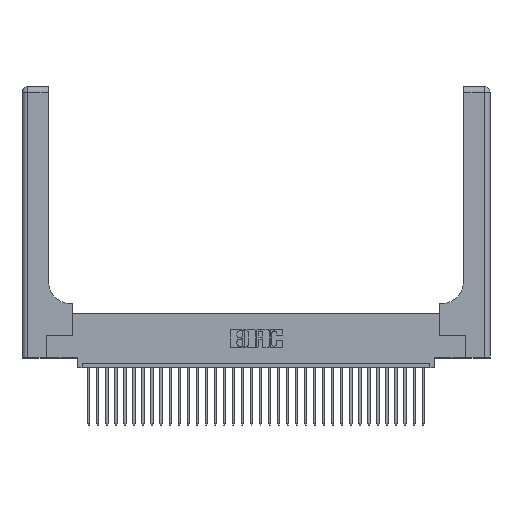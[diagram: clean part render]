
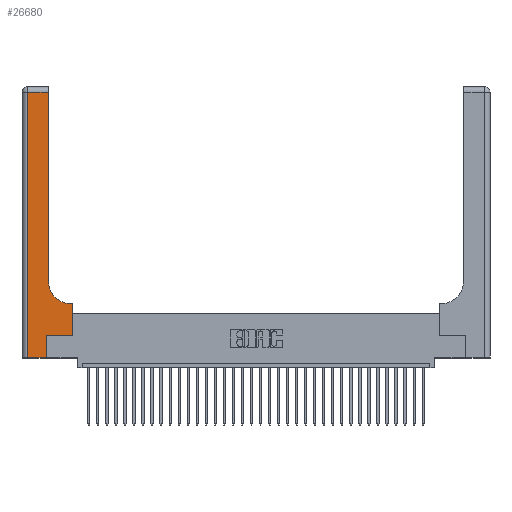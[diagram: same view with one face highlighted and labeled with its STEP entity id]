
A CAD part, top view. The second image highlights one B-rep face of the part: STEP entity #26680.
In plain terms, the highlighted planar face has unit normal (0, 0, 1).
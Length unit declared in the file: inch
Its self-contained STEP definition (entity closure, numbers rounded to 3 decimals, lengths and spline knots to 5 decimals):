
#269 = ORIENTED_EDGE ( 'NONE', *, *, #11622, .T. ) ;
#581 = CARTESIAN_POINT ( 'NONE',  ( 0.2915, 0.85, 0.37 ) ) ;
#1344 = LINE ( 'NONE', #22579, #9231 ) ;
#1752 = VERTEX_POINT ( 'NONE', #25194 ) ;
#2163 = CARTESIAN_POINT ( 'NONE',  ( 0.2915, 3., 0.37 ) ) ;
#3003 = EDGE_CURVE ( 'NONE', #11323, #3056, #8525, .T. ) ;
#3056 = VERTEX_POINT ( 'NONE', #7794 ) ;
#3455 = CARTESIAN_POINT ( 'NONE',  ( 0.269, 0.25, 0.37 ) ) ;
#3712 = DIRECTION ( 'NONE',  ( 1., 0., 0. ) ) ;
#4756 = EDGE_CURVE ( 'NONE', #32752, #34467, #1344, .T. ) ;
#4982 = LINE ( 'NONE', #12663, #9131 ) ;
#5082 = CARTESIAN_POINT ( 'NONE',  ( 0.5415, 0.6, 0.37 ) ) ;
#5227 = VECTOR ( 'NONE', #7631, 39.37008 ) ;
#5939 = VECTOR ( 'NONE', #33972, 39.37008 ) ;
#6462 = CARTESIAN_POINT ( 'NONE',  ( 0.06, 0., 0.37 ) ) ;
#6854 = DIRECTION ( 'NONE',  ( 0., 0., -1. ) ) ;
#6968 = LINE ( 'NONE', #7161, #7808 ) ;
#7161 = CARTESIAN_POINT ( 'NONE',  ( 0.5585, 0.25, 0.37 ) ) ;
#7584 = CARTESIAN_POINT ( 'NONE',  ( 0.2915, 0.6, 0.37 ) ) ;
#7631 = DIRECTION ( 'NONE',  ( 1., 0., 0. ) ) ;
#7659 = LINE ( 'NONE', #7584, #5939 ) ;
#7794 = CARTESIAN_POINT ( 'NONE',  ( 0.269, 0., 0.37 ) ) ;
#7808 = VECTOR ( 'NONE', #12409, 39.37008 ) ;
#8030 = ORIENTED_EDGE ( 'NONE', *, *, #11778, .T. ) ;
#8525 = LINE ( 'NONE', #12889, #5227 ) ;
#8648 = EDGE_CURVE ( 'NONE', #1752, #29394, #6968, .T. ) ;
#9131 = VECTOR ( 'NONE', #25964, 39.37008 ) ;
#9231 = VECTOR ( 'NONE', #12066, 39.37008 ) ;
#11323 = VERTEX_POINT ( 'NONE', #6462 ) ;
#11380 = VECTOR ( 'NONE', #23519, 39.37008 ) ;
#11572 = CIRCLE ( 'NONE', #15827, 0.25 ) ;
#11622 = EDGE_CURVE ( 'NONE', #31362, #32752, #12240, .T. ) ;
#11778 = EDGE_CURVE ( 'NONE', #29394, #23675, #7659, .T. ) ;
#11857 = LINE ( 'NONE', #15061, #16799 ) ;
#12066 = DIRECTION ( 'NONE',  ( -1., 0., 0. ) ) ;
#12240 = LINE ( 'NONE', #2163, #11380 ) ;
#12409 = DIRECTION ( 'NONE',  ( 0., 1., 0. ) ) ;
#12663 = CARTESIAN_POINT ( 'NONE',  ( 0.269, 0.25, 0.37 ) ) ;
#12860 = CARTESIAN_POINT ( 'NONE',  ( 0., 3., 0.37 ) ) ;
#12889 = CARTESIAN_POINT ( 'NONE',  ( 0., 0., 0.37 ) ) ;
#12910 = EDGE_CURVE ( 'NONE', #34396, #1752, #4982, .T. ) ;
#14344 = VECTOR ( 'NONE', #23931, 39.37008 ) ;
#15061 = CARTESIAN_POINT ( 'NONE',  ( 0.269, 0., 0.37 ) ) ;
#15827 = AXIS2_PLACEMENT_3D ( 'NONE', #22754, #6854, #3712 ) ;
#15978 = EDGE_CURVE ( 'NONE', #34467, #11323, #20129, .T. ) ;
#16799 = VECTOR ( 'NONE', #28039, 39.37008 ) ;
#17010 = FACE_OUTER_BOUND ( 'NONE', #18750, .T. ) ;
#17164 = ORIENTED_EDGE ( 'NONE', *, *, #27214, .T. ) ;
#18388 = PLANE ( 'NONE',  #26477 ) ;
#18750 = EDGE_LOOP ( 'NONE', ( #269, #23766, #33423, #32667, #19051, #28663, #31304, #8030, #17164 ) ) ;
#19051 = ORIENTED_EDGE ( 'NONE', *, *, #29310, .T. ) ;
#19373 = CARTESIAN_POINT ( 'NONE',  ( 0.06, 2.94, 0.37 ) ) ;
#20129 = LINE ( 'NONE', #21042, #14344 ) ;
#20729 = CARTESIAN_POINT ( 'NONE',  ( 0.5585, 0.6, 0.37 ) ) ;
#21042 = CARTESIAN_POINT ( 'NONE',  ( 0.06, 3., 0.37 ) ) ;
#22579 = CARTESIAN_POINT ( 'NONE',  ( 0., 2.94, 0.37 ) ) ;
#22754 = CARTESIAN_POINT ( 'NONE',  ( 0.5415, 0.85, 0.37 ) ) ;
#23519 = DIRECTION ( 'NONE',  ( 0., 1., 0. ) ) ;
#23675 = VERTEX_POINT ( 'NONE', #5082 ) ;
#23766 = ORIENTED_EDGE ( 'NONE', *, *, #4756, .T. ) ;
#23931 = DIRECTION ( 'NONE',  ( 0., -1., 0. ) ) ;
#25194 = CARTESIAN_POINT ( 'NONE',  ( 0.5585, 0.25, 0.37 ) ) ;
#25556 = CARTESIAN_POINT ( 'NONE',  ( 0.2915, 2.94, 0.37 ) ) ;
#25964 = DIRECTION ( 'NONE',  ( 1., 0., 0. ) ) ;
#26163 = DIRECTION ( 'NONE',  ( 0., 0., -1. ) ) ;
#26477 = AXIS2_PLACEMENT_3D ( 'NONE', #12860, #26163, #30815 ) ;
#26680 = ADVANCED_FACE ( 'NONE', ( #17010 ), #18388, .F. ) ;
#27214 = EDGE_CURVE ( 'NONE', #23675, #31362, #11572, .T. ) ;
#28039 = DIRECTION ( 'NONE',  ( 0., 1., 0. ) ) ;
#28663 = ORIENTED_EDGE ( 'NONE', *, *, #12910, .T. ) ;
#29310 = EDGE_CURVE ( 'NONE', #3056, #34396, #11857, .T. ) ;
#29394 = VERTEX_POINT ( 'NONE', #20729 ) ;
#30815 = DIRECTION ( 'NONE',  ( -1., 0., 0. ) ) ;
#31304 = ORIENTED_EDGE ( 'NONE', *, *, #8648, .T. ) ;
#31362 = VERTEX_POINT ( 'NONE', #581 ) ;
#32667 = ORIENTED_EDGE ( 'NONE', *, *, #3003, .T. ) ;
#32752 = VERTEX_POINT ( 'NONE', #25556 ) ;
#33423 = ORIENTED_EDGE ( 'NONE', *, *, #15978, .T. ) ;
#33972 = DIRECTION ( 'NONE',  ( -1., 0., 0. ) ) ;
#34396 = VERTEX_POINT ( 'NONE', #3455 ) ;
#34467 = VERTEX_POINT ( 'NONE', #19373 ) ;
